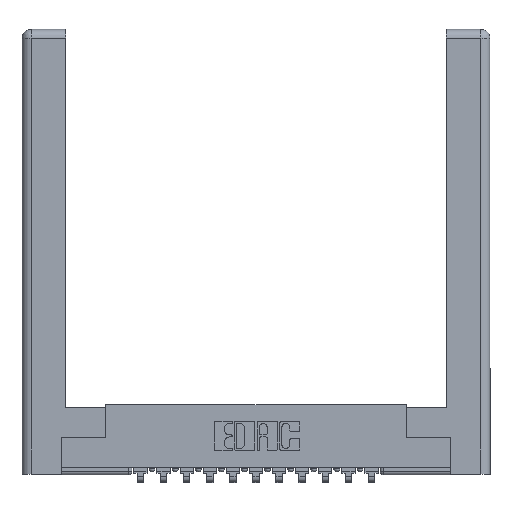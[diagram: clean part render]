
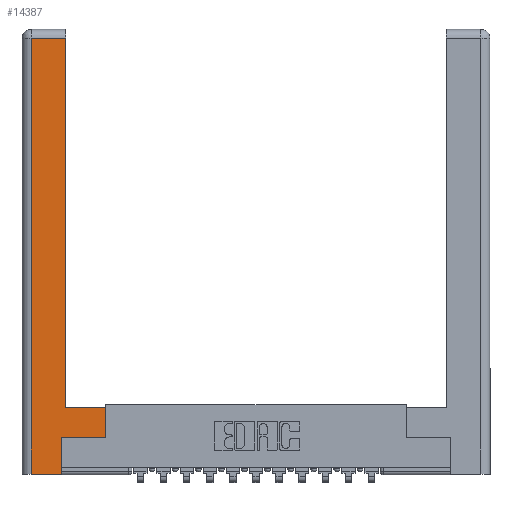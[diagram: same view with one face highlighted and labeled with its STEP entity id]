
A CAD part, top view. The second image highlights one B-rep face of the part: STEP entity #14387.
In plain terms, the highlighted planar face has unit normal (0, 0, 1).
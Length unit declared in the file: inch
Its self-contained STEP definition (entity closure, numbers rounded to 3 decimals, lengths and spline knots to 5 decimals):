
#174 = ORIENTED_EDGE ( 'NONE', *, *, #9648, .T. ) ;
#738 = CARTESIAN_POINT ( 'NONE',  ( 0.295, 3., 0. ) ) ;
#819 = CARTESIAN_POINT ( 'NONE',  ( 0.565, 0.245, 0. ) ) ;
#1034 = VERTEX_POINT ( 'NONE', #3973 ) ;
#1186 = DIRECTION ( 'NONE',  ( 0., 1., 0. ) ) ;
#1326 = ORIENTED_EDGE ( 'NONE', *, *, #14020, .T. ) ;
#1330 = EDGE_CURVE ( 'NONE', #15711, #1034, #14758, .T. ) ;
#1434 = EDGE_CURVE ( 'NONE', #15820, #15711, #4214, .T. ) ;
#2028 = VERTEX_POINT ( 'NONE', #4974 ) ;
#2577 = DIRECTION ( 'NONE',  ( 1., 0., 0. ) ) ;
#2738 = CARTESIAN_POINT ( 'NONE',  ( 0.295, 0.45, 0. ) ) ;
#2915 = CARTESIAN_POINT ( 'NONE',  ( 0.565, 0.245, 0. ) ) ;
#3220 = VECTOR ( 'NONE', #7146, 39.37008 ) ;
#3229 = ORIENTED_EDGE ( 'NONE', *, *, #6009, .T. ) ;
#3973 = CARTESIAN_POINT ( 'NONE',  ( 0.0615, 2.94, 0. ) ) ;
#4110 = DIRECTION ( 'NONE',  ( 0., -1., 0. ) ) ;
#4214 = LINE ( 'NONE', #738, #9276 ) ;
#4499 = CARTESIAN_POINT ( 'NONE',  ( 0.0615, 2.94, 0. ) ) ;
#4554 = LINE ( 'NONE', #4580, #8807 ) ;
#4580 = CARTESIAN_POINT ( 'NONE',  ( 0.265, 0.245, 0. ) ) ;
#4742 = DIRECTION ( 'NONE',  ( 1., 0., 0. ) ) ;
#4771 = DIRECTION ( 'NONE',  ( 0., 1., 0. ) ) ;
#4974 = CARTESIAN_POINT ( 'NONE',  ( 0.265, 0., 0. ) ) ;
#5448 = ORIENTED_EDGE ( 'NONE', *, *, #1330, .T. ) ;
#5845 = LINE ( 'NONE', #13116, #14161 ) ;
#5847 = ORIENTED_EDGE ( 'NONE', *, *, #1434, .T. ) ;
#5870 = CARTESIAN_POINT ( 'NONE',  ( 0.295, 2.94, 0. ) ) ;
#6009 = EDGE_CURVE ( 'NONE', #10478, #15820, #13597, .T. ) ;
#6210 = FACE_OUTER_BOUND ( 'NONE', #10409, .T. ) ;
#6225 = LINE ( 'NONE', #12936, #12739 ) ;
#6683 = VECTOR ( 'NONE', #10438, 39.37008 ) ;
#6725 = ORIENTED_EDGE ( 'NONE', *, *, #7381, .T. ) ;
#6960 = PLANE ( 'NONE',  #13287 ) ;
#7146 = DIRECTION ( 'NONE',  ( -1., 0., 0. ) ) ;
#7233 = LINE ( 'NONE', #8510, #14552 ) ;
#7381 = EDGE_CURVE ( 'NONE', #8443, #12546, #11105, .T. ) ;
#7623 = VECTOR ( 'NONE', #4742, 39.37008 ) ;
#8278 = CARTESIAN_POINT ( 'NONE',  ( 0.295, 0.45, 0. ) ) ;
#8443 = VERTEX_POINT ( 'NONE', #14226 ) ;
#8510 = CARTESIAN_POINT ( 'NONE',  ( 0.565, 0.45, 0. ) ) ;
#8807 = VECTOR ( 'NONE', #15969, 39.37008 ) ;
#9276 = VECTOR ( 'NONE', #1186, 39.37008 ) ;
#9613 = ORIENTED_EDGE ( 'NONE', *, *, #14289, .T. ) ;
#9648 = EDGE_CURVE ( 'NONE', #1034, #11996, #5845, .T. ) ;
#10409 = EDGE_LOOP ( 'NONE', ( #5847, #5448, #174, #9613, #15904, #6725, #1326, #3229 ) ) ;
#10438 = DIRECTION ( 'NONE',  ( -1., 0., 0. ) ) ;
#10478 = VERTEX_POINT ( 'NONE', #11165 ) ;
#10634 = CARTESIAN_POINT ( 'NONE',  ( 0.0615, 0., 0. ) ) ;
#11019 = DIRECTION ( 'NONE',  ( -1., 0., 0. ) ) ;
#11105 = LINE ( 'NONE', #819, #7623 ) ;
#11165 = CARTESIAN_POINT ( 'NONE',  ( 0.565, 0.45, 0. ) ) ;
#11996 = VERTEX_POINT ( 'NONE', #10634 ) ;
#12150 = CARTESIAN_POINT ( 'NONE',  ( 0., 0., 0. ) ) ;
#12546 = VERTEX_POINT ( 'NONE', #2915 ) ;
#12739 = VECTOR ( 'NONE', #2577, 39.37008 ) ;
#12936 = CARTESIAN_POINT ( 'NONE',  ( 0.265, 0., 0. ) ) ;
#13116 = CARTESIAN_POINT ( 'NONE',  ( 0.0615, 0., 0. ) ) ;
#13287 = AXIS2_PLACEMENT_3D ( 'NONE', #12150, #16038, #11019 ) ;
#13597 = LINE ( 'NONE', #2738, #6683 ) ;
#14020 = EDGE_CURVE ( 'NONE', #12546, #10478, #7233, .T. ) ;
#14161 = VECTOR ( 'NONE', #4110, 39.37008 ) ;
#14226 = CARTESIAN_POINT ( 'NONE',  ( 0.265, 0.245, 0. ) ) ;
#14289 = EDGE_CURVE ( 'NONE', #11996, #2028, #6225, .T. ) ;
#14387 = ADVANCED_FACE ( 'NONE', ( #6210 ), #6960, .F. ) ;
#14552 = VECTOR ( 'NONE', #4771, 39.37008 ) ;
#14758 = LINE ( 'NONE', #4499, #3220 ) ;
#15711 = VERTEX_POINT ( 'NONE', #5870 ) ;
#15803 = EDGE_CURVE ( 'NONE', #2028, #8443, #4554, .T. ) ;
#15820 = VERTEX_POINT ( 'NONE', #8278 ) ;
#15904 = ORIENTED_EDGE ( 'NONE', *, *, #15803, .T. ) ;
#15969 = DIRECTION ( 'NONE',  ( 0., 1., 0. ) ) ;
#16038 = DIRECTION ( 'NONE',  ( 0., 0., -1. ) ) ;
